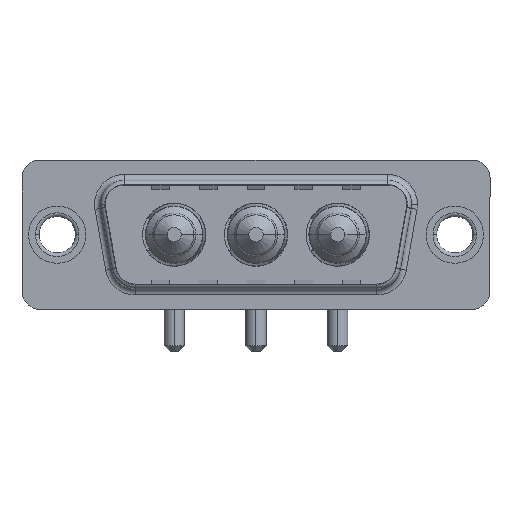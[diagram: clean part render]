
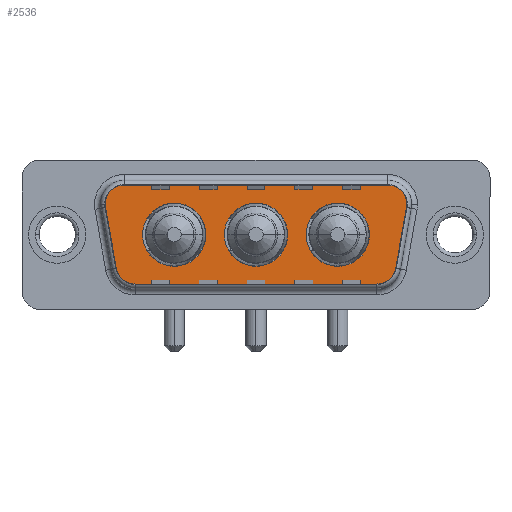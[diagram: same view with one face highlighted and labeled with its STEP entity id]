
A CAD part, top view. The second image highlights one B-rep face of the part: STEP entity #2536.
In plain terms, the highlighted planar face has unit normal (0, 0, 1).
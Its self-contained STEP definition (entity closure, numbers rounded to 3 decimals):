
#123 = ORIENTED_EDGE ( 'NONE', *, *, #3991, .T. ) ;
#163 = DIRECTION ( 'NONE',  ( 0., 0., 1. ) ) ;
#239 = AXIS2_PLACEMENT_3D ( 'NONE', #9796, #8165, #2769 ) ;
#480 = DIRECTION ( 'NONE',  ( 0., 0., 1. ) ) ;
#560 = EDGE_LOOP ( 'NONE', ( #6958, #1279 ) ) ;
#568 = CARTESIAN_POINT ( 'NONE',  ( 28.836, -3.247, 0. ) ) ;
#584 = CARTESIAN_POINT ( 'NONE',  ( 16.65, 0., 0. ) ) ;
#607 = VECTOR ( 'NONE', #6396, 1000. ) ;
#677 = CARTESIAN_POINT ( 'NONE',  ( 14., 0., 0. ) ) ;
#737 = AXIS2_PLACEMENT_3D ( 'NONE', #5085, #9570, #7824 ) ;
#748 = CIRCLE ( 'NONE', #239, 2. ) ;
#821 = CARTESIAN_POINT ( 'NONE',  ( 6.434, -4.9, 0. ) ) ;
#822 = EDGE_CURVE ( 'NONE', #3947, #3084, #10405, .T. ) ;
#906 = ORIENTED_EDGE ( 'NONE', *, *, #7573, .F. ) ;
#1019 = DIRECTION ( 'NONE',  ( 0., 0., 1. ) ) ;
#1072 = DIRECTION ( 'NONE',  ( 1., 0., 0. ) ) ;
#1196 = CIRCLE ( 'NONE', #7302, 2.65 ) ;
#1279 = ORIENTED_EDGE ( 'NONE', *, *, #10891, .F. ) ;
#1305 = CIRCLE ( 'NONE', #6158, 2. ) ;
#1517 = CARTESIAN_POINT ( 'NONE',  ( 4.464, -3.247, 0. ) ) ;
#1538 = CARTESIAN_POINT ( 'NONE',  ( 23.5, 0., 0. ) ) ;
#1583 = EDGE_CURVE ( 'NONE', #5492, #9165, #3994, .T. ) ;
#1818 = CARTESIAN_POINT ( 'NONE',  ( 26.866, -2.9, 0. ) ) ;
#2126 = CARTESIAN_POINT ( 'NONE',  ( 16.65, 0., 0. ) ) ;
#2135 = CARTESIAN_POINT ( 'NONE',  ( 5.411, 2.9, 0. ) ) ;
#2136 = DIRECTION ( 'NONE',  ( -1., 0., 0. ) ) ;
#2243 = VERTEX_POINT ( 'NONE', #10607 ) ;
#2389 = VECTOR ( 'NONE', #8117, 1000. ) ;
#2429 = DIRECTION ( 'NONE',  ( 0., 0., 1. ) ) ;
#2519 = AXIS2_PLACEMENT_3D ( 'NONE', #6338, #163, #9646 ) ;
#2536 = ADVANCED_FACE ( 'NONE', ( #6205, #6095, #7100, #3803 ), #2657, .T. ) ;
#2636 = CARTESIAN_POINT ( 'NONE',  ( 3.441, 2.553, 0. ) ) ;
#2641 = CARTESIAN_POINT ( 'NONE',  ( 9.8, 0., 0. ) ) ;
#2657 = PLANE ( 'NONE',  #9891 ) ;
#2769 = DIRECTION ( 'NONE',  ( -1., 0., 0. ) ) ;
#2968 = LINE ( 'NONE', #6449, #607 ) ;
#2995 = CARTESIAN_POINT ( 'NONE',  ( 27.889, 2.9, 0. ) ) ;
#3048 = DIRECTION ( 'NONE',  ( 0., 0., 1. ) ) ;
#3084 = VERTEX_POINT ( 'NONE', #568 ) ;
#3121 = EDGE_CURVE ( 'NONE', #8225, #3743, #1305, .T. ) ;
#3138 = AXIS2_PLACEMENT_3D ( 'NONE', #5916, #9283, #9338 ) ;
#3150 = DIRECTION ( 'NONE',  ( 0., 0., 1. ) ) ;
#3182 = CIRCLE ( 'NONE', #6409, 2.65 ) ;
#3273 = VERTEX_POINT ( 'NONE', #3437 ) ;
#3373 = ORIENTED_EDGE ( 'NONE', *, *, #822, .T. ) ;
#3391 = CARTESIAN_POINT ( 'NONE',  ( 12.45, 0., 0. ) ) ;
#3401 = VECTOR ( 'NONE', #9497, 1000. ) ;
#3437 = CARTESIAN_POINT ( 'NONE',  ( 29.889, 2.9, 0. ) ) ;
#3711 = CARTESIAN_POINT ( 'NONE',  ( 19.3, 0., 0. ) ) ;
#3743 = VERTEX_POINT ( 'NONE', #8637 ) ;
#3803 = FACE_OUTER_BOUND ( 'NONE', #7272, .T. ) ;
#3947 = VERTEX_POINT ( 'NONE', #10535 ) ;
#3985 = ORIENTED_EDGE ( 'NONE', *, *, #6791, .F. ) ;
#3991 = EDGE_CURVE ( 'NONE', #2243, #8225, #2968, .T. ) ;
#3994 = CIRCLE ( 'NONE', #5957, 2.65 ) ;
#4029 = DIRECTION ( 'NONE',  ( 1., 0., 0. ) ) ;
#4116 = AXIS2_PLACEMENT_3D ( 'NONE', #2126, #3150, #6578 ) ;
#4196 = CARTESIAN_POINT ( 'NONE',  ( 20.85, 0., 0. ) ) ;
#4202 = CARTESIAN_POINT ( 'NONE',  ( 29.859, 2.553, 0. ) ) ;
#4308 = VERTEX_POINT ( 'NONE', #677 ) ;
#4410 = EDGE_CURVE ( 'NONE', #6875, #5003, #5112, .T. ) ;
#4516 = CARTESIAN_POINT ( 'NONE',  ( 6.434, -4.9, 0. ) ) ;
#4610 = VERTEX_POINT ( 'NONE', #821 ) ;
#4657 = CIRCLE ( 'NONE', #4116, 2.65 ) ;
#4872 = CIRCLE ( 'NONE', #8446, 2.65 ) ;
#4950 = ORIENTED_EDGE ( 'NONE', *, *, #8598, .T. ) ;
#5003 = VERTEX_POINT ( 'NONE', #10092 ) ;
#5085 = CARTESIAN_POINT ( 'NONE',  ( 27.889, 2.9, 0. ) ) ;
#5101 = ORIENTED_EDGE ( 'NONE', *, *, #7491, .T. ) ;
#5112 = CIRCLE ( 'NONE', #3138, 2.65 ) ;
#5300 = LINE ( 'NONE', #4516, #9852 ) ;
#5336 = EDGE_LOOP ( 'NONE', ( #906, #3985 ) ) ;
#5433 = CIRCLE ( 'NONE', #737, 2. ) ;
#5492 = VERTEX_POINT ( 'NONE', #3391 ) ;
#5516 = AXIS2_PLACEMENT_3D ( 'NONE', #2995, #6420, #2136 ) ;
#5647 = LINE ( 'NONE', #7206, #2389 ) ;
#5815 = DIRECTION ( 'NONE',  ( 1., 0., 0. ) ) ;
#5884 = ORIENTED_EDGE ( 'NONE', *, *, #4410, .F. ) ;
#5916 = CARTESIAN_POINT ( 'NONE',  ( 23.5, 0., 0. ) ) ;
#5918 = EDGE_CURVE ( 'NONE', #3273, #2243, #10694, .T. ) ;
#5957 = AXIS2_PLACEMENT_3D ( 'NONE', #10074, #2429, #5815 ) ;
#6046 = ORIENTED_EDGE ( 'NONE', *, *, #8384, .T. ) ;
#6095 = FACE_BOUND ( 'NONE', #7231, .T. ) ;
#6147 = VERTEX_POINT ( 'NONE', #3711 ) ;
#6158 = AXIS2_PLACEMENT_3D ( 'NONE', #2135, #3048, #6476 ) ;
#6205 = FACE_BOUND ( 'NONE', #5336, .T. ) ;
#6269 = EDGE_CURVE ( 'NONE', #5003, #6875, #3182, .T. ) ;
#6338 = CARTESIAN_POINT ( 'NONE',  ( 26.866, -2.9, 0. ) ) ;
#6374 = ORIENTED_EDGE ( 'NONE', *, *, #8176, .T. ) ;
#6396 = DIRECTION ( 'NONE',  ( -1., 0., 0. ) ) ;
#6409 = AXIS2_PLACEMENT_3D ( 'NONE', #1538, #9198, #9251 ) ;
#6420 = DIRECTION ( 'NONE',  ( 0., 0., 1. ) ) ;
#6449 = CARTESIAN_POINT ( 'NONE',  ( 5.411, 4.9, 0. ) ) ;
#6476 = DIRECTION ( 'NONE',  ( 1., 0., 0. ) ) ;
#6578 = DIRECTION ( 'NONE',  ( 1., 0., 0. ) ) ;
#6791 = EDGE_CURVE ( 'NONE', #4308, #6147, #1196, .T. ) ;
#6875 = VERTEX_POINT ( 'NONE', #4196 ) ;
#6958 = ORIENTED_EDGE ( 'NONE', *, *, #1583, .F. ) ;
#7032 = DIRECTION ( 'NONE',  ( 0., 0., 1. ) ) ;
#7100 = FACE_BOUND ( 'NONE', #560, .T. ) ;
#7206 = CARTESIAN_POINT ( 'NONE',  ( 29.859, 2.553, 0. ) ) ;
#7231 = EDGE_LOOP ( 'NONE', ( #8953, #5884 ) ) ;
#7272 = EDGE_LOOP ( 'NONE', ( #3373, #9430, #6374, #10884, #123, #9354, #4950, #6046, #5101 ) ) ;
#7302 = AXIS2_PLACEMENT_3D ( 'NONE', #584, #480, #4029 ) ;
#7491 = EDGE_CURVE ( 'NONE', #4610, #3947, #5300, .T. ) ;
#7573 = EDGE_CURVE ( 'NONE', #6147, #4308, #4657, .T. ) ;
#7824 = DIRECTION ( 'NONE',  ( -1., 0., 0. ) ) ;
#8117 = DIRECTION ( 'NONE',  ( 0.174, 0.985, 0. ) ) ;
#8165 = DIRECTION ( 'NONE',  ( 0., 0., 1. ) ) ;
#8176 = EDGE_CURVE ( 'NONE', #9115, #3273, #5433, .T. ) ;
#8225 = VERTEX_POINT ( 'NONE', #8722 ) ;
#8384 = EDGE_CURVE ( 'NONE', #8477, #4610, #748, .T. ) ;
#8446 = AXIS2_PLACEMENT_3D ( 'NONE', #2641, #7032, #10390 ) ;
#8477 = VERTEX_POINT ( 'NONE', #1517 ) ;
#8598 = EDGE_CURVE ( 'NONE', #3743, #8477, #11017, .T. ) ;
#8637 = CARTESIAN_POINT ( 'NONE',  ( 3.441, 2.553, 0. ) ) ;
#8722 = CARTESIAN_POINT ( 'NONE',  ( 5.411, 4.9, 0. ) ) ;
#8953 = ORIENTED_EDGE ( 'NONE', *, *, #6269, .F. ) ;
#9115 = VERTEX_POINT ( 'NONE', #4202 ) ;
#9165 = VERTEX_POINT ( 'NONE', #9629 ) ;
#9198 = DIRECTION ( 'NONE',  ( 0., 0., 1. ) ) ;
#9251 = DIRECTION ( 'NONE',  ( 1., 0., 0. ) ) ;
#9283 = DIRECTION ( 'NONE',  ( 0., 0., 1. ) ) ;
#9337 = EDGE_CURVE ( 'NONE', #3084, #9115, #5647, .T. ) ;
#9338 = DIRECTION ( 'NONE',  ( 1., 0., 0. ) ) ;
#9354 = ORIENTED_EDGE ( 'NONE', *, *, #3121, .T. ) ;
#9430 = ORIENTED_EDGE ( 'NONE', *, *, #9337, .T. ) ;
#9497 = DIRECTION ( 'NONE',  ( 0.174, -0.985, 0. ) ) ;
#9554 = DIRECTION ( 'NONE',  ( 1., 0., 0. ) ) ;
#9570 = DIRECTION ( 'NONE',  ( 0., 0., 1. ) ) ;
#9629 = CARTESIAN_POINT ( 'NONE',  ( 7.15, 0., 0. ) ) ;
#9646 = DIRECTION ( 'NONE',  ( 1., 0., 0. ) ) ;
#9796 = CARTESIAN_POINT ( 'NONE',  ( 6.434, -2.9, 0. ) ) ;
#9852 = VECTOR ( 'NONE', #9554, 1000. ) ;
#9891 = AXIS2_PLACEMENT_3D ( 'NONE', #1818, #1019, #1072 ) ;
#10074 = CARTESIAN_POINT ( 'NONE',  ( 9.8, 0., 0. ) ) ;
#10092 = CARTESIAN_POINT ( 'NONE',  ( 26.15, 0., 0. ) ) ;
#10390 = DIRECTION ( 'NONE',  ( 1., 0., 0. ) ) ;
#10405 = CIRCLE ( 'NONE', #2519, 2. ) ;
#10535 = CARTESIAN_POINT ( 'NONE',  ( 26.866, -4.9, 0. ) ) ;
#10607 = CARTESIAN_POINT ( 'NONE',  ( 27.889, 4.9, 0. ) ) ;
#10694 = CIRCLE ( 'NONE', #5516, 2. ) ;
#10884 = ORIENTED_EDGE ( 'NONE', *, *, #5918, .T. ) ;
#10891 = EDGE_CURVE ( 'NONE', #9165, #5492, #4872, .T. ) ;
#11017 = LINE ( 'NONE', #2636, #3401 ) ;
